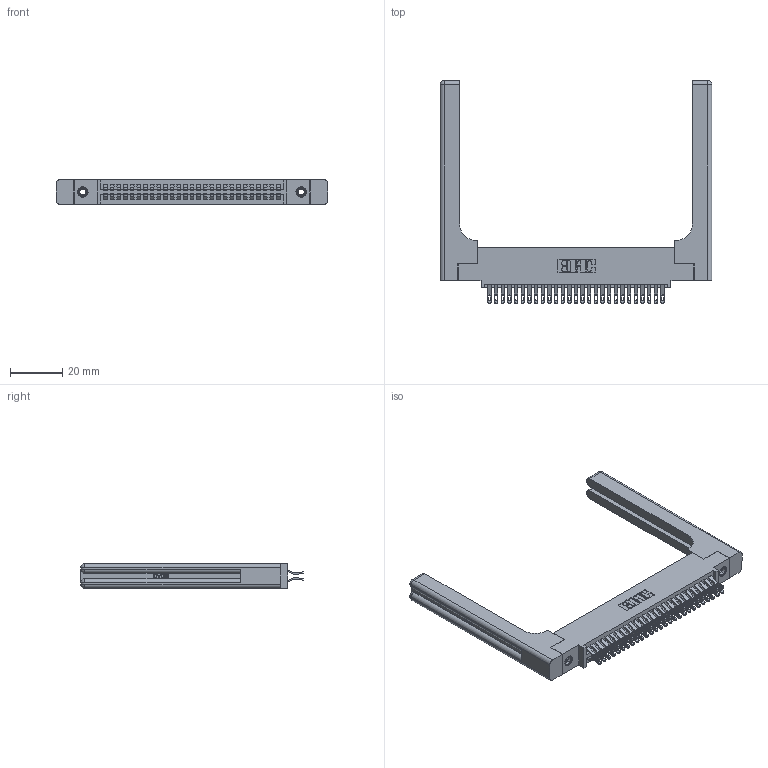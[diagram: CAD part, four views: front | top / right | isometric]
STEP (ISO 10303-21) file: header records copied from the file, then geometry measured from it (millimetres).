
FILE_DESCRIPTION (( 'STEP AP203' ), '1' );
FILE_NAME ('345-054-555-558.STEP', '2019-10-29T19:40:38', ( '' ), ( '' ), 'SwSTEP 2.0', 'SolidWorks 2016', '' );
FILE_SCHEMA (( 'CONFIG_CONTROL_DESIGN' ));
Length unit declared in the file: inch
Products named in the file (5): 345-054-555-558; 345-250-001_345-250-001-102; 345-220-058_345-220-058; 345-292-001_555 Tail; 345 Part_0.110 Offset - 0.156 Dia-TH
Assembly tree (59 placements, depth 2):
  345-054-555-558
    345 Part_0.110 Offset - 0.156 Dia-TH
    345-292-001_555 Tail  x54
    345-250-001_345-250-001-102  x2
    345-220-058_345-220-058  x2
Bounding box: 103.61 x 84.89 x 9.4 mm (x, y, z)
Volume: 18483.6 mm3; surface area: 20200.2 mm2
Topology: 59 solids, 59 shells, 3410 faces, 10577 edges, 7030 vertices
Faces by surface type: plane 1906, cylinder 1444, bspline 36, cone 12, sphere 8, torus 4
Entity records: 28844 total; most frequent: CARTESIAN_POINT 5879, ORIENTED_EDGE 4580, DIRECTION 4102, EDGE_CURVE 2290, LINE 1938, VECTOR 1938, VERTEX_POINT 1518, AXIS2_PLACEMENT_3D 1082
